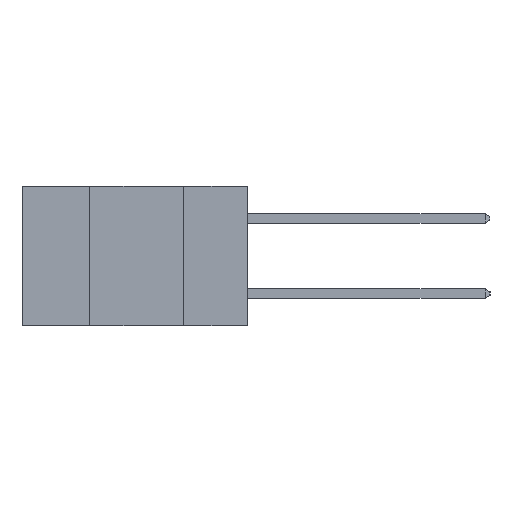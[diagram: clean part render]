
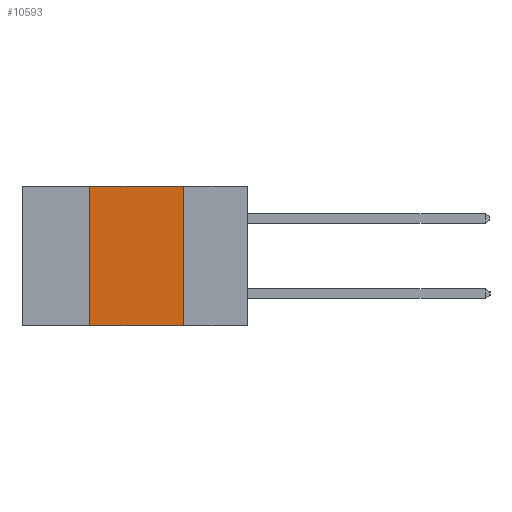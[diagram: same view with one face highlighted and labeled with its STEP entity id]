
A CAD part, left-side view. The second image highlights one B-rep face of the part: STEP entity #10593.
In plain terms, the highlighted planar face has unit normal (-1, 0, 0).
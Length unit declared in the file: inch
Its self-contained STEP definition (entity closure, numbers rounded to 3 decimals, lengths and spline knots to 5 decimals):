
#11 = VECTOR ( 'NONE', #12868, 39.37008 ) ;
#598 = CARTESIAN_POINT ( 'NONE',  ( 0., 0.6, 0. ) ) ;
#842 = CARTESIAN_POINT ( 'NONE',  ( 0., 0.17, 0. ) ) ;
#920 = VECTOR ( 'NONE', #7925, 39.37008 ) ;
#1014 = CARTESIAN_POINT ( 'NONE',  ( 0., 0.17, -0.37 ) ) ;
#1611 = ORIENTED_EDGE ( 'NONE', *, *, #17880, .F. ) ;
#1708 = ORIENTED_EDGE ( 'NONE', *, *, #13706, .F. ) ;
#1862 = VERTEX_POINT ( 'NONE', #842 ) ;
#2031 = ORIENTED_EDGE ( 'NONE', *, *, #16543, .T. ) ;
#2340 = ORIENTED_EDGE ( 'NONE', *, *, #17425, .F. ) ;
#2456 = DIRECTION ( 'NONE',  ( 0., 0., -1. ) ) ;
#3326 = LINE ( 'NONE', #1014, #7579 ) ;
#3453 = DIRECTION ( 'NONE',  ( 1., 0., 0. ) ) ;
#3794 = LINE ( 'NONE', #16789, #11 ) ;
#4410 = CARTESIAN_POINT ( 'NONE',  ( 0., 0.6, 0. ) ) ;
#5483 = CARTESIAN_POINT ( 'NONE',  ( 0., 0.17, -0.37 ) ) ;
#6085 = LINE ( 'NONE', #6519, #920 ) ;
#6448 = CARTESIAN_POINT ( 'NONE',  ( 0., 0.42, 0. ) ) ;
#6519 = CARTESIAN_POINT ( 'NONE',  ( 0., 0.6, -0.37 ) ) ;
#7542 = VERTEX_POINT ( 'NONE', #6448 ) ;
#7579 = VECTOR ( 'NONE', #2456, 39.37008 ) ;
#7651 = VERTEX_POINT ( 'NONE', #5483 ) ;
#7925 = DIRECTION ( 'NONE',  ( 0., -1., 0. ) ) ;
#8718 = EDGE_LOOP ( 'NONE', ( #1611, #1708, #2340, #2031 ) ) ;
#9371 = CARTESIAN_POINT ( 'NONE',  ( 0., 0.42, -0.37 ) ) ;
#10593 = ADVANCED_FACE ( 'NONE', ( #17122 ), #15936, .F. ) ;
#10759 = VECTOR ( 'NONE', #14237, 39.37008 ) ;
#12762 = AXIS2_PLACEMENT_3D ( 'NONE', #598, #3453, #13336 ) ;
#12868 = DIRECTION ( 'NONE',  ( 0., 0., 1. ) ) ;
#13336 = DIRECTION ( 'NONE',  ( 0., 0., -1. ) ) ;
#13706 = EDGE_CURVE ( 'NONE', #7542, #1862, #14395, .T. ) ;
#14237 = DIRECTION ( 'NONE',  ( 0., -1., 0. ) ) ;
#14395 = LINE ( 'NONE', #4410, #10759 ) ;
#15936 = PLANE ( 'NONE',  #12762 ) ;
#16543 = EDGE_CURVE ( 'NONE', #16549, #7651, #6085, .T. ) ;
#16549 = VERTEX_POINT ( 'NONE', #9371 ) ;
#16789 = CARTESIAN_POINT ( 'NONE',  ( 0., 0.42, -0.37 ) ) ;
#17122 = FACE_OUTER_BOUND ( 'NONE', #8718, .T. ) ;
#17425 = EDGE_CURVE ( 'NONE', #16549, #7542, #3794, .T. ) ;
#17880 = EDGE_CURVE ( 'NONE', #1862, #7651, #3326, .T. ) ;
